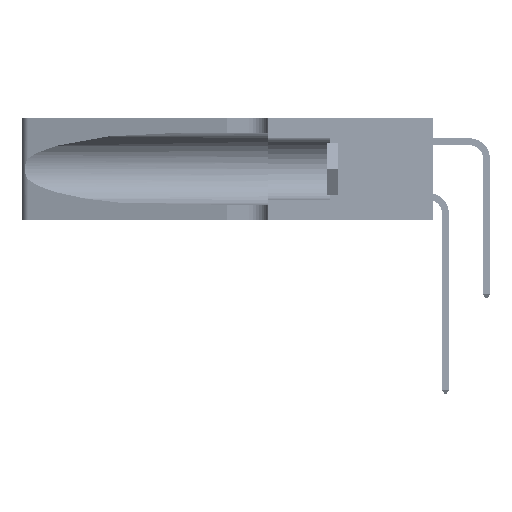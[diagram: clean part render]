
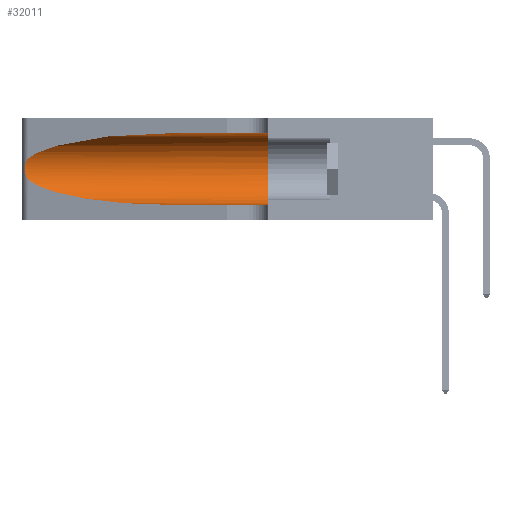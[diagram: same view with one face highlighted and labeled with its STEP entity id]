
A CAD part, left-side view. The second image highlights one B-rep face of the part: STEP entity #32011.
In plain terms, the highlighted cylindrical face has radius 3.308 mm (diameter 6.617 mm), a partial arc.
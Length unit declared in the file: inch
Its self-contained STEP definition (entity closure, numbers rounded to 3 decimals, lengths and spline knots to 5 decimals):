
#532 = CARTESIAN_POINT ( 'NONE',  ( 0.25487, 1.22718, 0.22369 ) ) ;
#722 = CARTESIAN_POINT ( 'NONE',  ( 0.25487, 1.22718, 0.22369 ) ) ;
#900 = CARTESIAN_POINT ( 'NONE',  ( 0.26075, 1.23896, 0.178 ) ) ;
#1084 = FACE_OUTER_BOUND ( 'NONE', #5349, .T. ) ;
#1652 = CARTESIAN_POINT ( 'NONE',  ( 0.1305, 1.61858, 0.185 ) ) ;
#2705 = EDGE_CURVE ( 'NONE', #22087, #8938, #50126, .T. ) ;
#3507 = VECTOR ( 'NONE', #8925, 39.37008 ) ;
#4674 = CARTESIAN_POINT ( 'NONE',  ( 0.1305, 1.61858, 0.31525 ) ) ;
#5155 = CARTESIAN_POINT ( 'NONE',  ( 0.25856, 1.23593, 0.16098 ) ) ;
#5241 = CARTESIAN_POINT ( 'NONE',  ( 0.25487, 1.22718, 0.14631 ) ) ;
#5349 = EDGE_LOOP ( 'NONE', ( #48916, #20174, #30127, #20518, #51481, #45065 ) ) ;
#6024 = VERTEX_POINT ( 'NONE', #29453 ) ;
#6062 = EDGE_CURVE ( 'NONE', #13300, #6024, #36275, .T. ) ;
#8925 = DIRECTION ( 'NONE',  ( 0., -1., 0. ) ) ;
#8938 = VERTEX_POINT ( 'NONE', #53697 ) ;
#9042 = EDGE_CURVE ( 'NONE', #30781, #6024, #38230, .T. ) ;
#9409 = CARTESIAN_POINT ( 'NONE',  ( 0.25639, 1.23186, 0.15144 ) ) ;
#10803 = CARTESIAN_POINT ( 'NONE',  ( 0.1305, 0.72297, 0.31525 ) ) ;
#12433 = DIRECTION ( 'NONE',  ( 0., -1., 0. ) ) ;
#12690 = DIRECTION ( 'NONE',  ( 0., 1., 0. ) ) ;
#13110 = CARTESIAN_POINT ( 'NONE',  ( 0.1305, 0.72297, 0.31525 ) ) ;
#13300 = VERTEX_POINT ( 'NONE', #50785 ) ;
#13654 = CARTESIAN_POINT ( 'NONE',  ( 0.25487, 1.22718, 0.14631 ) ) ;
#13735 = CARTESIAN_POINT ( 'NONE',  ( 0.1305, 0.72297, 0.05475 ) ) ;
#14222 = DIRECTION ( 'NONE',  ( 0., 0., -1. ) ) ;
#17087 = EDGE_CURVE ( 'NONE', #37317, #30781, #44206, .T. ) ;
#17695 = CARTESIAN_POINT ( 'NONE',  ( 0.25639, 1.23184, 0.21858 ) ) ;
#17978 =( BOUNDED_CURVE ( )  B_SPLINE_CURVE ( 3, ( #5241, #30372, #38777, #13735 ),
 .UNSPECIFIED., .F., .F. ) 
 B_SPLINE_CURVE_WITH_KNOTS ( ( 4, 4 ),
 ( 3.44316, 4.71239 ),
 .UNSPECIFIED. ) 
 CURVE ( )  GEOMETRIC_REPRESENTATION_ITEM ( )  RATIONAL_B_SPLINE_CURVE ( ( 1., 0.87, 0.87, 1. ) ) 
 REPRESENTATION_ITEM ( '' )  );
#18287 =( BOUNDED_CURVE ( )  B_SPLINE_CURVE ( 3, ( #13110, #46568, #25694, #532 ),
 .UNSPECIFIED., .F., .F. ) 
 B_SPLINE_CURVE_WITH_KNOTS ( ( 4, 4 ),
 ( 1.5708, 2.84003 ),
 .UNSPECIFIED. ) 
 CURVE ( )  GEOMETRIC_REPRESENTATION_ITEM ( )  RATIONAL_B_SPLINE_CURVE ( ( 1., 0.87, 0.87, 1. ) ) 
 REPRESENTATION_ITEM ( '' )  );
#20174 = ORIENTED_EDGE ( 'NONE', *, *, #2705, .T. ) ;
#20518 = ORIENTED_EDGE ( 'NONE', *, *, #6062, .T. ) ;
#21874 = CARTESIAN_POINT ( 'NONE',  ( 0.25854, 1.2359, 0.20912 ) ) ;
#22087 = VERTEX_POINT ( 'NONE', #46118 ) ;
#25694 = CARTESIAN_POINT ( 'NONE',  ( 0.2373, 1.15595, 0.28018 ) ) ;
#26072 = CARTESIAN_POINT ( 'NONE',  ( 0.26075, 1.23896, 0.19203 ) ) ;
#26716 = AXIS2_PLACEMENT_3D ( 'NONE', #1652, #51925, #14222 ) ;
#28415 = EDGE_CURVE ( 'NONE', #8938, #13300, #17978, .T. ) ;
#29453 = CARTESIAN_POINT ( 'NONE',  ( 0.1305, 0.35, 0.05475 ) ) ;
#30127 = ORIENTED_EDGE ( 'NONE', *, *, #28415, .T. ) ;
#30287 = CARTESIAN_POINT ( 'NONE',  ( 0.26017, 1.23833, 0.17102 ) ) ;
#30372 = CARTESIAN_POINT ( 'NONE',  ( 0.2373, 1.15595, 0.08982 ) ) ;
#30781 = VERTEX_POINT ( 'NONE', #47604 ) ;
#32011 = ADVANCED_FACE ( 'NONE', ( #1084 ), #33240, .F. ) ;
#32339 = VECTOR ( 'NONE', #12433, 39.37008 ) ;
#33240 = CYLINDRICAL_SURFACE ( 'NONE', #26716, 0.13025 ) ;
#34456 = CARTESIAN_POINT ( 'NONE',  ( 0.25789, 1.23486, 0.15765 ) ) ;
#36275 = LINE ( 'NONE', #37307, #32339 ) ;
#37307 = CARTESIAN_POINT ( 'NONE',  ( 0.1305, 1.61858, 0.05475 ) ) ;
#37317 = VERTEX_POINT ( 'NONE', #10803 ) ;
#37715 = CARTESIAN_POINT ( 'NONE',  ( 0.1305, 0.35, 0.185 ) ) ;
#38230 = CIRCLE ( 'NONE', #48303, 0.13025 ) ;
#38695 = CARTESIAN_POINT ( 'NONE',  ( 0.25555, 1.22993, 0.14849 ) ) ;
#38777 = CARTESIAN_POINT ( 'NONE',  ( 0.18966, 0.96281, 0.05475 ) ) ;
#41965 = DIRECTION ( 'NONE',  ( 0., 0., 1. ) ) ;
#42733 = CARTESIAN_POINT ( 'NONE',  ( 0.25555, 1.22994, 0.2215 ) ) ;
#44206 = LINE ( 'NONE', #4674, #3507 ) ;
#45065 = ORIENTED_EDGE ( 'NONE', *, *, #17087, .F. ) ;
#46118 = CARTESIAN_POINT ( 'NONE',  ( 0.25487, 1.22718, 0.22369 ) ) ;
#46568 = CARTESIAN_POINT ( 'NONE',  ( 0.18966, 0.96281, 0.31525 ) ) ;
#46952 = CARTESIAN_POINT ( 'NONE',  ( 0.25787, 1.23484, 0.2124 ) ) ;
#47604 = CARTESIAN_POINT ( 'NONE',  ( 0.1305, 0.35, 0.31525 ) ) ;
#48303 = AXIS2_PLACEMENT_3D ( 'NONE', #37715, #12690, #41965 ) ;
#48916 = ORIENTED_EDGE ( 'NONE', *, *, #52546, .T. ) ;
#50126 = B_SPLINE_CURVE_WITH_KNOTS ( 'NONE', 3,
 ( #722, #42733, #17695, #46952, #21874, #51172, #26072, #900, #30287, #5155, #34456, #9409, #38695, #13654 ),
 .UNSPECIFIED., .F., .F.,
 ( 4, 2, 2, 2, 2, 2, 4 ),
 ( 0., 0.00027, 0.00053, 0.00107, 0.0016, 0.00187, 0.00214 ),
 .UNSPECIFIED. ) ;
#50785 = CARTESIAN_POINT ( 'NONE',  ( 0.1305, 0.72297, 0.05475 ) ) ;
#51172 = CARTESIAN_POINT ( 'NONE',  ( 0.26018, 1.23835, 0.19895 ) ) ;
#51481 = ORIENTED_EDGE ( 'NONE', *, *, #9042, .F. ) ;
#51925 = DIRECTION ( 'NONE',  ( 0., -1., 0. ) ) ;
#52546 = EDGE_CURVE ( 'NONE', #37317, #22087, #18287, .T. ) ;
#53697 = CARTESIAN_POINT ( 'NONE',  ( 0.25487, 1.22718, 0.14631 ) ) ;
